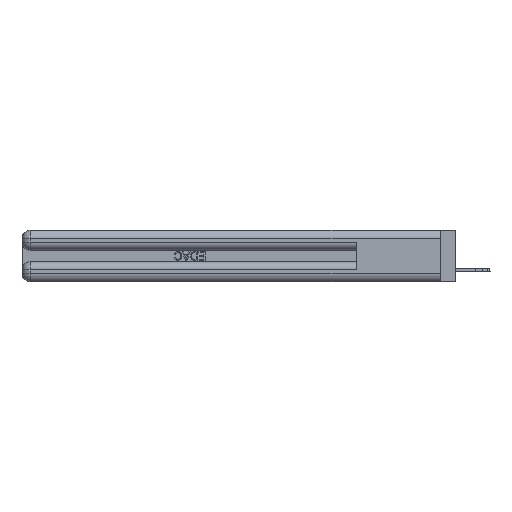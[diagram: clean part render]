
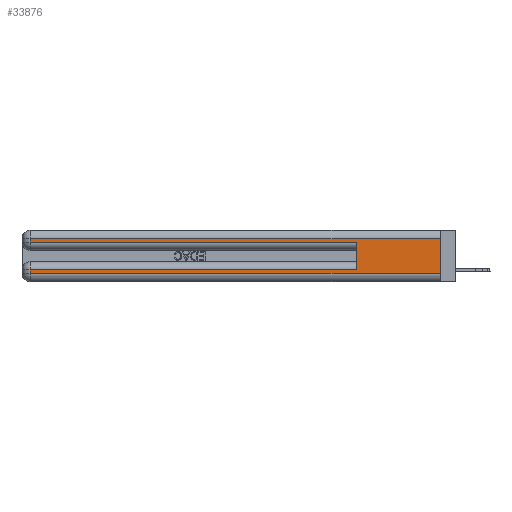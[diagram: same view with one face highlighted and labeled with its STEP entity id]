
A CAD part, left-side view. The second image highlights one B-rep face of the part: STEP entity #33876.
In plain terms, the highlighted planar face has unit normal (-1, 0, 0).
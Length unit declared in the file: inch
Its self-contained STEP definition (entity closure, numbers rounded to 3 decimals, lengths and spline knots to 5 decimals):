
#307 = PLANE ( 'NONE',  #36889 ) ;
#415 = DIRECTION ( 'NONE',  ( 0., 0., -1. ) ) ;
#1934 = LINE ( 'NONE', #14872, #17480 ) ;
#2476 = CARTESIAN_POINT ( 'NONE',  ( 0., 0., 0.31 ) ) ;
#2897 = LINE ( 'NONE', #12287, #34603 ) ;
#3310 = LINE ( 'NONE', #33068, #11572 ) ;
#3720 = CARTESIAN_POINT ( 'NONE',  ( 0., 2.94, 0.085 ) ) ;
#3908 = VERTEX_POINT ( 'NONE', #11324 ) ;
#4469 = DIRECTION ( 'NONE',  ( 0., -1., 0. ) ) ;
#5029 = CARTESIAN_POINT ( 'NONE',  ( 0., 0., 0.06 ) ) ;
#5215 = DIRECTION ( 'NONE',  ( 0., 1., 0. ) ) ;
#5397 = ORIENTED_EDGE ( 'NONE', *, *, #29580, .F. ) ;
#6214 = VECTOR ( 'NONE', #5215, 39.37008 ) ;
#7666 = CARTESIAN_POINT ( 'NONE',  ( 0., 0.6, 0.085 ) ) ;
#8377 = VECTOR ( 'NONE', #12353, 39.37008 ) ;
#8786 = VERTEX_POINT ( 'NONE', #9749 ) ;
#9560 = EDGE_CURVE ( 'NONE', #26859, #35318, #14048, .T. ) ;
#9749 = CARTESIAN_POINT ( 'NONE',  ( 0., 0.6, 0.285 ) ) ;
#10260 = VECTOR ( 'NONE', #34697, 39.37008 ) ;
#10667 = ORIENTED_EDGE ( 'NONE', *, *, #13215, .T. ) ;
#10822 = ORIENTED_EDGE ( 'NONE', *, *, #17543, .F. ) ;
#11324 = CARTESIAN_POINT ( 'NONE',  ( 0., 2.94, 0.06 ) ) ;
#11572 = VECTOR ( 'NONE', #26755, 39.37008 ) ;
#12287 = CARTESIAN_POINT ( 'NONE',  ( 0., 2.94, 0.37 ) ) ;
#12353 = DIRECTION ( 'NONE',  ( 0., 0., 1. ) ) ;
#12481 = EDGE_CURVE ( 'NONE', #21519, #3908, #2897, .T. ) ;
#13215 = EDGE_CURVE ( 'NONE', #19550, #8786, #1934, .T. ) ;
#13856 = EDGE_CURVE ( 'NONE', #3908, #28682, #16974, .T. ) ;
#14048 = LINE ( 'NONE', #22836, #6214 ) ;
#14647 = DIRECTION ( 'NONE',  ( 1., 0., 0. ) ) ;
#14872 = CARTESIAN_POINT ( 'NONE',  ( 0., 0., 0.285 ) ) ;
#16974 = LINE ( 'NONE', #22019, #24836 ) ;
#17480 = VECTOR ( 'NONE', #35481, 39.37008 ) ;
#17543 = EDGE_CURVE ( 'NONE', #26859, #28682, #35635, .T. ) ;
#19550 = VERTEX_POINT ( 'NONE', #36070 ) ;
#21519 = VERTEX_POINT ( 'NONE', #3720 ) ;
#21927 = DIRECTION ( 'NONE',  ( 0., 0., -1. ) ) ;
#22019 = CARTESIAN_POINT ( 'NONE',  ( 0., 0., 0.06 ) ) ;
#22187 = EDGE_LOOP ( 'NONE', ( #10822, #26503, #32776, #10667, #5397, #36129, #36950, #33359 ) ) ;
#22836 = CARTESIAN_POINT ( 'NONE',  ( 0., 0., 0.31 ) ) ;
#22988 = CARTESIAN_POINT ( 'NONE',  ( 0., 2.94, 0.37 ) ) ;
#23434 = FACE_OUTER_BOUND ( 'NONE', #22187, .T. ) ;
#24183 = EDGE_CURVE ( 'NONE', #35318, #19550, #33751, .T. ) ;
#24836 = VECTOR ( 'NONE', #4469, 39.37008 ) ;
#26503 = ORIENTED_EDGE ( 'NONE', *, *, #9560, .T. ) ;
#26755 = DIRECTION ( 'NONE',  ( 0., 1., 0. ) ) ;
#26859 = VERTEX_POINT ( 'NONE', #2476 ) ;
#28415 = CARTESIAN_POINT ( 'NONE',  ( 0., 2.94, 0.31 ) ) ;
#28682 = VERTEX_POINT ( 'NONE', #5029 ) ;
#29580 = EDGE_CURVE ( 'NONE', #31113, #8786, #37471, .T. ) ;
#29962 = CARTESIAN_POINT ( 'NONE',  ( 0., 0.6, 0.145 ) ) ;
#30227 = EDGE_CURVE ( 'NONE', #31113, #21519, #3310, .T. ) ;
#31113 = VERTEX_POINT ( 'NONE', #7666 ) ;
#32776 = ORIENTED_EDGE ( 'NONE', *, *, #24183, .T. ) ;
#32790 = CARTESIAN_POINT ( 'NONE',  ( 0., 0., 0.37 ) ) ;
#33010 = CARTESIAN_POINT ( 'NONE',  ( 0., 0., 0.37 ) ) ;
#33068 = CARTESIAN_POINT ( 'NONE',  ( 0., 0., 0.085 ) ) ;
#33359 = ORIENTED_EDGE ( 'NONE', *, *, #13856, .T. ) ;
#33751 = LINE ( 'NONE', #22988, #10260 ) ;
#33814 = VECTOR ( 'NONE', #21927, 39.37008 ) ;
#33876 = ADVANCED_FACE ( 'NONE', ( #23434 ), #307, .F. ) ;
#34603 = VECTOR ( 'NONE', #415, 39.37008 ) ;
#34697 = DIRECTION ( 'NONE',  ( 0., 0., -1. ) ) ;
#35269 = DIRECTION ( 'NONE',  ( 0., 0., -1. ) ) ;
#35318 = VERTEX_POINT ( 'NONE', #28415 ) ;
#35481 = DIRECTION ( 'NONE',  ( 0., -1., 0. ) ) ;
#35635 = LINE ( 'NONE', #33010, #33814 ) ;
#36070 = CARTESIAN_POINT ( 'NONE',  ( 0., 2.94, 0.285 ) ) ;
#36129 = ORIENTED_EDGE ( 'NONE', *, *, #30227, .T. ) ;
#36889 = AXIS2_PLACEMENT_3D ( 'NONE', #32790, #14647, #35269 ) ;
#36950 = ORIENTED_EDGE ( 'NONE', *, *, #12481, .T. ) ;
#37471 = LINE ( 'NONE', #29962, #8377 ) ;
